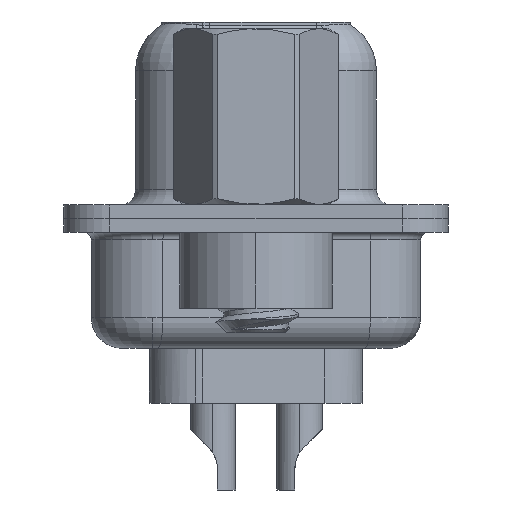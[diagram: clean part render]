
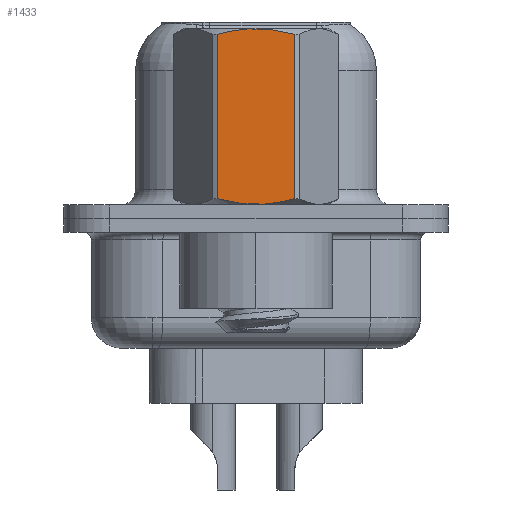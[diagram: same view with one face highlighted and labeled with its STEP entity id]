
A CAD part, left-side view. The second image highlights one B-rep face of the part: STEP entity #1433.
In plain terms, the highlighted planar face has unit normal (-1, 0, 0).
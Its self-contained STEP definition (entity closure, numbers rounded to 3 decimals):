
#11 = PLANE ( 'NONE',  #7341 ) ;
#530 = ORIENTED_EDGE ( 'NONE', *, *, #8982, .T. ) ;
#1429 = CARTESIAN_POINT ( 'NONE',  ( -2.381, 1.273, 0.652 ) ) ;
#1433 = ADVANCED_FACE ( 'NONE', ( #23396 ), #11, .T. ) ;
#1670 = CARTESIAN_POINT ( 'NONE',  ( -2.381, -0.215, 6.232 ) ) ;
#1821 = CARTESIAN_POINT ( 'NONE',  ( -2.381, 1.273, 0.652 ) ) ;
#2256 = CARTESIAN_POINT ( 'NONE',  ( -2.381, -0.858, 6.15 ) ) ;
#3167 = CARTESIAN_POINT ( 'NONE',  ( -2.381, -1.273, 0.652 ) ) ;
#3178 = VERTEX_POINT ( 'NONE', #3167 ) ;
#3812 = LINE ( 'NONE', #8277, #20450 ) ;
#4023 = CARTESIAN_POINT ( 'NONE',  ( -2.381, -1.066, 0.596 ) ) ;
#4110 = CARTESIAN_POINT ( 'NONE',  ( -2.381, 0.428, 6.215 ) ) ;
#4899 = CARTESIAN_POINT ( 'NONE',  ( -2.381, 1.375, -3.75 ) ) ;
#5279 = DIRECTION ( 'NONE',  ( 0., 0., 1. ) ) ;
#5737 = LINE ( 'NONE', #7897, #15814 ) ;
#6020 = B_SPLINE_CURVE_WITH_KNOTS ( 'NONE', 3,
 ( #1429, #29427, #13226, #8488, #27108, #15516, #8629, #15662, #4023, #7225 ),
 .UNSPECIFIED., .F., .F.,
 ( 4, 2, 2, 2, 4 ),
 ( 0.003, 0.003, 0.004, 0.004, 0.005 ),
 .UNSPECIFIED. ) ;
#6830 = EDGE_CURVE ( 'NONE', #8625, #21208, #3812, .T. ) ;
#7225 = CARTESIAN_POINT ( 'NONE',  ( -2.381, -1.273, 0.652 ) ) ;
#7341 = AXIS2_PLACEMENT_3D ( 'NONE', #4899, #21121, #16694 ) ;
#7897 = CARTESIAN_POINT ( 'NONE',  ( -2.381, -1.273, 3.792 ) ) ;
#8138 = VERTEX_POINT ( 'NONE', #9960 ) ;
#8277 = CARTESIAN_POINT ( 'NONE',  ( -2.381, 1.273, 3.792 ) ) ;
#8488 = CARTESIAN_POINT ( 'NONE',  ( -2.381, 0.428, 0.485 ) ) ;
#8625 = VERTEX_POINT ( 'NONE', #15053 ) ;
#8629 = CARTESIAN_POINT ( 'NONE',  ( -2.381, -0.432, 0.485 ) ) ;
#8982 = EDGE_CURVE ( 'NONE', #8138, #8625, #27452, .T. ) ;
#9960 = CARTESIAN_POINT ( 'NONE',  ( -2.381, -1.273, 6.048 ) ) ;
#11008 = CARTESIAN_POINT ( 'NONE',  ( -2.381, 0.215, 6.232 ) ) ;
#13226 = CARTESIAN_POINT ( 'NONE',  ( -2.381, 0.853, 0.549 ) ) ;
#13460 = CARTESIAN_POINT ( 'NONE',  ( -2.381, 0.853, 6.151 ) ) ;
#15053 = CARTESIAN_POINT ( 'NONE',  ( -2.381, 1.273, 6.048 ) ) ;
#15383 = ORIENTED_EDGE ( 'NONE', *, *, #22812, .T. ) ;
#15516 = CARTESIAN_POINT ( 'NONE',  ( -2.381, -0.215, 0.468 ) ) ;
#15601 = CARTESIAN_POINT ( 'NONE',  ( -2.381, -0.432, 6.215 ) ) ;
#15662 = CARTESIAN_POINT ( 'NONE',  ( -2.381, -0.858, 0.55 ) ) ;
#15814 = VECTOR ( 'NONE', #5279, 1000. ) ;
#16694 = DIRECTION ( 'NONE',  ( 0., -1., 0. ) ) ;
#18202 = CARTESIAN_POINT ( 'NONE',  ( -2.381, -1.066, 6.104 ) ) ;
#18927 = ORIENTED_EDGE ( 'NONE', *, *, #25149, .T. ) ;
#20450 = VECTOR ( 'NONE', #22475, 1000. ) ;
#20813 = EDGE_LOOP ( 'NONE', ( #18927, #15383, #530, #21273 ) ) ;
#21121 = DIRECTION ( 'NONE',  ( -1., 0., 0. ) ) ;
#21208 = VERTEX_POINT ( 'NONE', #1821 ) ;
#21273 = ORIENTED_EDGE ( 'NONE', *, *, #6830, .T. ) ;
#21361 = CARTESIAN_POINT ( 'NONE',  ( -2.381, 1.273, 6.048 ) ) ;
#22475 = DIRECTION ( 'NONE',  ( 0., 0., -1. ) ) ;
#22812 = EDGE_CURVE ( 'NONE', #3178, #8138, #5737, .T. ) ;
#23216 = CARTESIAN_POINT ( 'NONE',  ( -2.381, -1.273, 6.048 ) ) ;
#23396 = FACE_OUTER_BOUND ( 'NONE', #20813, .T. ) ;
#25149 = EDGE_CURVE ( 'NONE', #21208, #3178, #6020, .T. ) ;
#27108 = CARTESIAN_POINT ( 'NONE',  ( -2.381, 0.215, 0.468 ) ) ;
#27452 = B_SPLINE_CURVE_WITH_KNOTS ( 'NONE', 3,
 ( #23216, #18202, #2256, #15601, #1670, #11008, #4110, #13460, #29819, #21361 ),
 .UNSPECIFIED., .F., .F.,
 ( 4, 2, 2, 2, 4 ),
 ( 0.001, 0.002, 0.002, 0.003, 0.004 ),
 .UNSPECIFIED. ) ;
#29427 = CARTESIAN_POINT ( 'NONE',  ( -2.381, 1.065, 0.596 ) ) ;
#29819 = CARTESIAN_POINT ( 'NONE',  ( -2.381, 1.065, 6.104 ) ) ;
